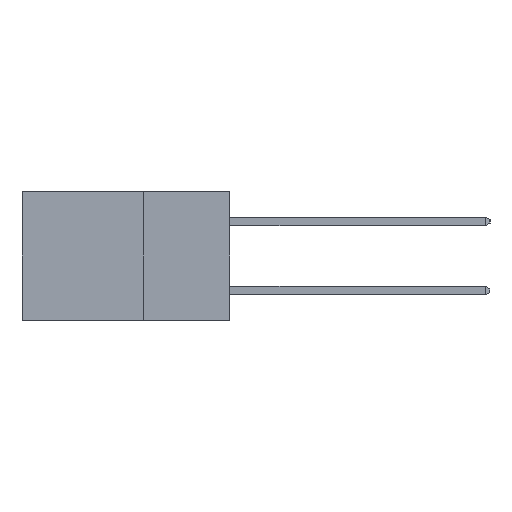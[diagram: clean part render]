
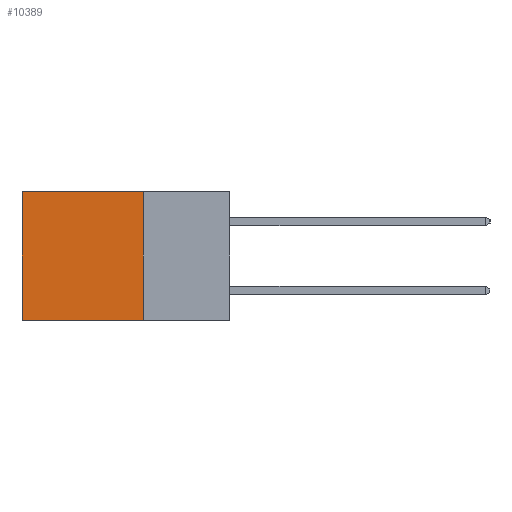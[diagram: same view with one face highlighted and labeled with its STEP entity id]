
A CAD part, left-side view. The second image highlights one B-rep face of the part: STEP entity #10389.
In plain terms, the highlighted planar face has unit normal (-1, 0, 0).
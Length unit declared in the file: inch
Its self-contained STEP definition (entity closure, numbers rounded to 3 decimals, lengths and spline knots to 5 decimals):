
#1168 = CARTESIAN_POINT ( 'NONE',  ( 0.298, 0.25, 0. ) ) ;
#2091 = LINE ( 'NONE', #19631, #11540 ) ;
#2782 = VECTOR ( 'NONE', #16923, 39.37008 ) ;
#2791 = LINE ( 'NONE', #1168, #20288 ) ;
#3012 = ORIENTED_EDGE ( 'NONE', *, *, #13686, .F. ) ;
#3690 = ORIENTED_EDGE ( 'NONE', *, *, #17196, .T. ) ;
#3753 = CARTESIAN_POINT ( 'NONE',  ( 0.298, 0.25, -0.37 ) ) ;
#4334 = PLANE ( 'NONE',  #14338 ) ;
#4644 = CARTESIAN_POINT ( 'NONE',  ( 0.298, 0.25, 0. ) ) ;
#5005 = VECTOR ( 'NONE', #13154, 39.37008 ) ;
#6116 = DIRECTION ( 'NONE',  ( 1., 0., 0. ) ) ;
#6221 = VERTEX_POINT ( 'NONE', #3753 ) ;
#8734 = CARTESIAN_POINT ( 'NONE',  ( 0.298, 0.6, 0. ) ) ;
#9292 = DIRECTION ( 'NONE',  ( 0., 1., 0. ) ) ;
#9579 = VERTEX_POINT ( 'NONE', #10719 ) ;
#9764 = LINE ( 'NONE', #18262, #5005 ) ;
#10389 = ADVANCED_FACE ( 'NONE', ( #16685 ), #4334, .F. ) ;
#10719 = CARTESIAN_POINT ( 'NONE',  ( 0.298, 0.25, 0. ) ) ;
#11540 = VECTOR ( 'NONE', #9292, 39.37008 ) ;
#11595 = ORIENTED_EDGE ( 'NONE', *, *, #22296, .T. ) ;
#11664 = LINE ( 'NONE', #4644, #2782 ) ;
#13138 = CARTESIAN_POINT ( 'NONE',  ( 0.298, 0.25, 0. ) ) ;
#13154 = DIRECTION ( 'NONE',  ( 0., 0., -1. ) ) ;
#13686 = EDGE_CURVE ( 'NONE', #6221, #20697, #2091, .T. ) ;
#14064 = EDGE_LOOP ( 'NONE', ( #11595, #3012, #22152, #3690 ) ) ;
#14338 = AXIS2_PLACEMENT_3D ( 'NONE', #13138, #6116, #18312 ) ;
#16685 = FACE_OUTER_BOUND ( 'NONE', #14064, .T. ) ;
#16923 = DIRECTION ( 'NONE',  ( 0., 0., -1. ) ) ;
#17196 = EDGE_CURVE ( 'NONE', #9579, #19367, #2791, .T. ) ;
#17585 = CARTESIAN_POINT ( 'NONE',  ( 0.298, 0.6, -0.37 ) ) ;
#18262 = CARTESIAN_POINT ( 'NONE',  ( 0.298, 0.6, 0. ) ) ;
#18312 = DIRECTION ( 'NONE',  ( 0., 0., -1. ) ) ;
#18631 = DIRECTION ( 'NONE',  ( 0., 1., 0. ) ) ;
#19367 = VERTEX_POINT ( 'NONE', #8734 ) ;
#19631 = CARTESIAN_POINT ( 'NONE',  ( 0.298, 0.25, -0.37 ) ) ;
#20288 = VECTOR ( 'NONE', #18631, 39.37008 ) ;
#20697 = VERTEX_POINT ( 'NONE', #17585 ) ;
#22152 = ORIENTED_EDGE ( 'NONE', *, *, #22427, .F. ) ;
#22296 = EDGE_CURVE ( 'NONE', #19367, #20697, #9764, .T. ) ;
#22427 = EDGE_CURVE ( 'NONE', #9579, #6221, #11664, .T. ) ;
